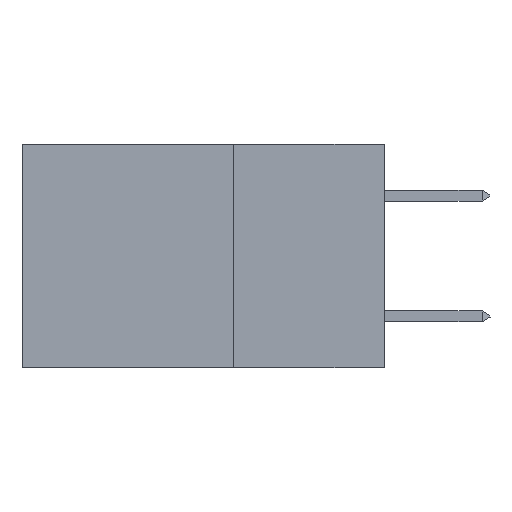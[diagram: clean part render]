
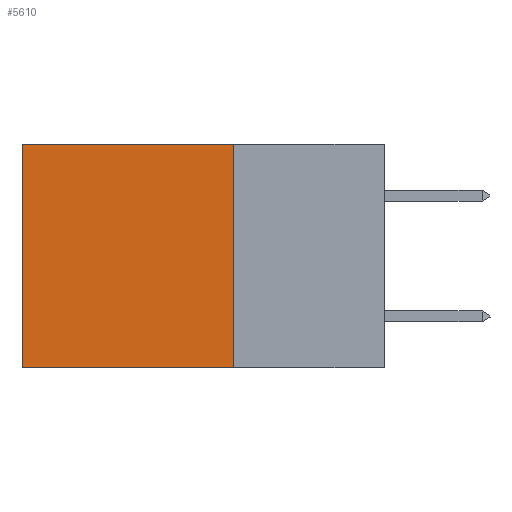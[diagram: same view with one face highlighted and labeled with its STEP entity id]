
A CAD part, left-side view. The second image highlights one B-rep face of the part: STEP entity #5610.
In plain terms, the highlighted planar face has unit normal (-1, 0, 0).
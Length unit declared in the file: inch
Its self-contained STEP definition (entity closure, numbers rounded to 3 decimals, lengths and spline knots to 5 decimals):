
#2636 = VECTOR ( 'NONE', #9571, 39.37008 ) ;
#4335 = VERTEX_POINT ( 'NONE', #27633 ) ;
#5179 = ORIENTED_EDGE ( 'NONE', *, *, #26423, .T. ) ;
#5245 = VECTOR ( 'NONE', #9821, 39.37008 ) ;
#5610 = ADVANCED_FACE ( 'NONE', ( #16771 ), #28070, .F. ) ;
#6322 = CARTESIAN_POINT ( 'NONE',  ( 0.2875, 0.25, 0. ) ) ;
#6995 = VECTOR ( 'NONE', #8464, 39.37008 ) ;
#7891 = CARTESIAN_POINT ( 'NONE',  ( 0.2875, 0.6, 0. ) ) ;
#8464 = DIRECTION ( 'NONE',  ( 0., 0., -1. ) ) ;
#9571 = DIRECTION ( 'NONE',  ( 0., 1., 0. ) ) ;
#9720 = CARTESIAN_POINT ( 'NONE',  ( 0.2875, 0.6, 0. ) ) ;
#9821 = DIRECTION ( 'NONE',  ( 0., 0., -1. ) ) ;
#10784 = ORIENTED_EDGE ( 'NONE', *, *, #21504, .T. ) ;
#10836 = DIRECTION ( 'NONE',  ( 1., 0., 0. ) ) ;
#11229 = LINE ( 'NONE', #9720, #5245 ) ;
#11956 = EDGE_CURVE ( 'NONE', #13792, #4335, #24500, .T. ) ;
#12531 = DIRECTION ( 'NONE',  ( 0., 1., 0. ) ) ;
#12863 = LINE ( 'NONE', #21506, #6995 ) ;
#13792 = VERTEX_POINT ( 'NONE', #15056 ) ;
#15056 = CARTESIAN_POINT ( 'NONE',  ( 0.2875, 0.25, -0.37 ) ) ;
#15176 = ORIENTED_EDGE ( 'NONE', *, *, #16905, .F. ) ;
#16750 = VERTEX_POINT ( 'NONE', #7891 ) ;
#16771 = FACE_OUTER_BOUND ( 'NONE', #18334, .T. ) ;
#16905 = EDGE_CURVE ( 'NONE', #19909, #13792, #12863, .T. ) ;
#17343 = VECTOR ( 'NONE', #12531, 39.37008 ) ;
#18334 = EDGE_LOOP ( 'NONE', ( #10784, #23824, #15176, #5179 ) ) ;
#19909 = VERTEX_POINT ( 'NONE', #28095 ) ;
#21504 = EDGE_CURVE ( 'NONE', #16750, #4335, #11229, .T. ) ;
#21506 = CARTESIAN_POINT ( 'NONE',  ( 0.2875, 0.25, 0. ) ) ;
#23066 = AXIS2_PLACEMENT_3D ( 'NONE', #6322, #10836, #26071 ) ;
#23362 = CARTESIAN_POINT ( 'NONE',  ( 0.2875, 0.25, -0.37 ) ) ;
#23824 = ORIENTED_EDGE ( 'NONE', *, *, #11956, .F. ) ;
#24500 = LINE ( 'NONE', #23362, #17343 ) ;
#24823 = CARTESIAN_POINT ( 'NONE',  ( 0.2875, 0.25, 0. ) ) ;
#26071 = DIRECTION ( 'NONE',  ( 0., 0., -1. ) ) ;
#26108 = LINE ( 'NONE', #24823, #2636 ) ;
#26423 = EDGE_CURVE ( 'NONE', #19909, #16750, #26108, .T. ) ;
#27633 = CARTESIAN_POINT ( 'NONE',  ( 0.2875, 0.6, -0.37 ) ) ;
#28070 = PLANE ( 'NONE',  #23066 ) ;
#28095 = CARTESIAN_POINT ( 'NONE',  ( 0.2875, 0.25, 0. ) ) ;
